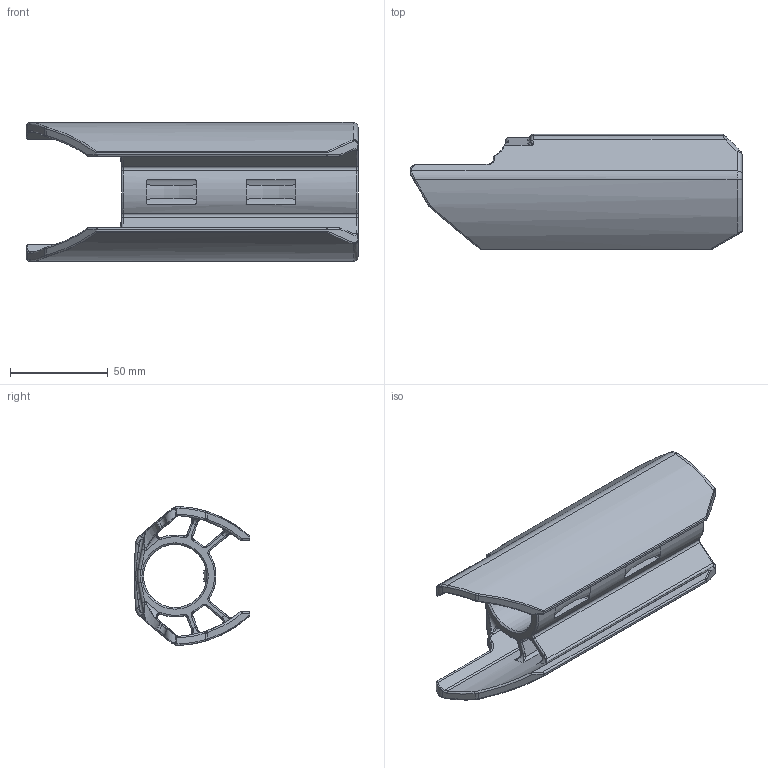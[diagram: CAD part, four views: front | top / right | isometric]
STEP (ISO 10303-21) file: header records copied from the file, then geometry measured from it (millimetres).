
FILE_DESCRIPTION (( 'STEP AP214' ), '1' );
FILE_NAME ('Pistol_Cheek_Rest.STEP', '2016-02-16T20:07:45', ( 'WarFairy' ), ( '' ), 'SwSTEP 2.0', 'SolidWorks 2015', '' );
FILE_SCHEMA (( 'AUTOMOTIVE_DESIGN' ));
Length unit declared in the file: inch
Products named in the file (1): Pistol_Cheek_Rest
Bounding box: 169.49 x 58.99 x 70.96 mm (x, y, z)
Volume: 183834.7 mm3; surface area: 73959.2 mm2
Topology: 1 solids, 1 shells, 369 faces, 919 edges, 521 vertices
Faces by surface type: cylinder 121, bspline 118, torus 72, plane 49, sphere 8, cone 1
Full cylindrical faces by diameter (mm): 32.258 x1
Entity records: 15177 total; most frequent: CARTESIAN_POINT 7607, ORIENTED_EDGE 1772, DIRECTION 1254, EDGE_CURVE 886, VERTEX_POINT 516, AXIS2_PLACEMENT_3D 513, EDGE_LOOP 384, FACE_OUTER_BOUND 370
